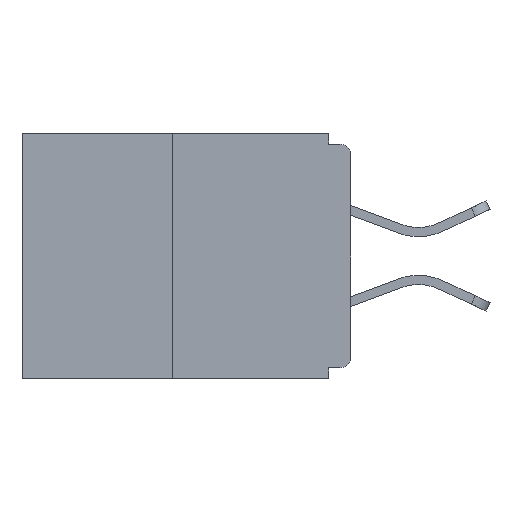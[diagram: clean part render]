
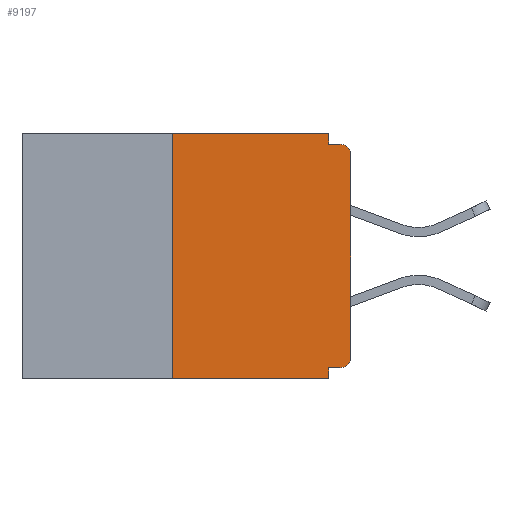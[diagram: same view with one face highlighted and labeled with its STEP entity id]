
A CAD part, left-side view. The second image highlights one B-rep face of the part: STEP entity #9197.
In plain terms, the highlighted planar face has unit normal (-1, 0, 0).
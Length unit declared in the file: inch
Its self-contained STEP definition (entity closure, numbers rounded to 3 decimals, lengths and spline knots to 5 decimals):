
#2 = VECTOR ( 'NONE', #19721, 39.37008 ) ;
#694 = DIRECTION ( 'NONE',  ( 0., 0., -1. ) ) ;
#788 = CARTESIAN_POINT ( 'NONE',  ( 0., 0.015, -0.03 ) ) ;
#896 = DIRECTION ( 'NONE',  ( 0., -1., 0. ) ) ;
#991 = VERTEX_POINT ( 'NONE', #12643 ) ;
#1147 = VERTEX_POINT ( 'NONE', #2009 ) ;
#1850 = LINE ( 'NONE', #9322, #15192 ) ;
#2009 = CARTESIAN_POINT ( 'NONE',  ( 0., 0., -0.313 ) ) ;
#2202 = VECTOR ( 'NONE', #11956, 39.37008 ) ;
#2434 = CIRCLE ( 'NONE', #19159, 0.015 ) ;
#2631 = EDGE_LOOP ( 'NONE', ( #3485, #15340, #22657, #20175, #4663, #16789, #5242, #20409, #9876, #16859 ) ) ;
#2703 = CARTESIAN_POINT ( 'NONE',  ( 0., 0., -0.015 ) ) ;
#2939 = CARTESIAN_POINT ( 'NONE',  ( 0., 0.031, -0.328 ) ) ;
#3423 = EDGE_CURVE ( 'NONE', #17848, #17363, #1850, .T. ) ;
#3485 = ORIENTED_EDGE ( 'NONE', *, *, #9588, .F. ) ;
#4242 = CIRCLE ( 'NONE', #18661, 0.015 ) ;
#4546 = VECTOR ( 'NONE', #11085, 39.37008 ) ;
#4663 = ORIENTED_EDGE ( 'NONE', *, *, #13185, .F. ) ;
#5237 = EDGE_CURVE ( 'NONE', #8949, #17363, #11205, .T. ) ;
#5242 = ORIENTED_EDGE ( 'NONE', *, *, #16992, .T. ) ;
#5782 = LINE ( 'NONE', #10197, #16762 ) ;
#6923 = VECTOR ( 'NONE', #18237, 39.37008 ) ;
#6983 = DIRECTION ( 'NONE',  ( 0., 1., 0. ) ) ;
#7072 = VERTEX_POINT ( 'NONE', #23327 ) ;
#7224 = LINE ( 'NONE', #10923, #19122 ) ;
#7410 = EDGE_CURVE ( 'NONE', #7072, #12155, #2434, .T. ) ;
#7433 = CARTESIAN_POINT ( 'NONE',  ( 0., 0.25, 0. ) ) ;
#8226 = DIRECTION ( 'NONE',  ( -1., 0., 0. ) ) ;
#8374 = CARTESIAN_POINT ( 'NONE',  ( 0., 0.46, 0. ) ) ;
#8459 = EDGE_CURVE ( 'NONE', #991, #12155, #19389, .T. ) ;
#8869 = EDGE_CURVE ( 'NONE', #16412, #1147, #4242, .T. ) ;
#8911 = EDGE_CURVE ( 'NONE', #8949, #9071, #23619, .T. ) ;
#8949 = VERTEX_POINT ( 'NONE', #10281 ) ;
#9071 = VERTEX_POINT ( 'NONE', #7433 ) ;
#9197 = ADVANCED_FACE ( 'NONE', ( #17611 ), #13836, .F. ) ;
#9322 = CARTESIAN_POINT ( 'NONE',  ( 0., 0.031, -0.343 ) ) ;
#9373 = LINE ( 'NONE', #12889, #6923 ) ;
#9588 = EDGE_CURVE ( 'NONE', #9071, #14831, #5782, .T. ) ;
#9646 = CARTESIAN_POINT ( 'NONE',  ( 0., 0.031, -0.343 ) ) ;
#9876 = ORIENTED_EDGE ( 'NONE', *, *, #8459, .F. ) ;
#9958 = DIRECTION ( 'NONE',  ( 0., -1., 0. ) ) ;
#10197 = CARTESIAN_POINT ( 'NONE',  ( 0., 0.46, 0. ) ) ;
#10281 = CARTESIAN_POINT ( 'NONE',  ( 0., 0.25, -0.343 ) ) ;
#10387 = CARTESIAN_POINT ( 'NONE',  ( 0., 0., 0. ) ) ;
#10553 = AXIS2_PLACEMENT_3D ( 'NONE', #8374, #21355, #694 ) ;
#10923 = CARTESIAN_POINT ( 'NONE',  ( 0., 0., -0.328 ) ) ;
#11085 = DIRECTION ( 'NONE',  ( 0., -1., 0. ) ) ;
#11205 = LINE ( 'NONE', #13130, #4546 ) ;
#11379 = DIRECTION ( 'NONE',  ( 0., 0., -1. ) ) ;
#11956 = DIRECTION ( 'NONE',  ( 0., 0., 1. ) ) ;
#12044 = VECTOR ( 'NONE', #896, 39.37008 ) ;
#12155 = VERTEX_POINT ( 'NONE', #18155 ) ;
#12643 = CARTESIAN_POINT ( 'NONE',  ( 0., 0.031, -0.015 ) ) ;
#12889 = CARTESIAN_POINT ( 'NONE',  ( 0., 0.031, 0. ) ) ;
#13130 = CARTESIAN_POINT ( 'NONE',  ( 0., 0.46, -0.343 ) ) ;
#13185 = EDGE_CURVE ( 'NONE', #16412, #17848, #7224, .T. ) ;
#13420 = CARTESIAN_POINT ( 'NONE',  ( 0., 0.015, -0.313 ) ) ;
#13836 = PLANE ( 'NONE',  #10553 ) ;
#14831 = VERTEX_POINT ( 'NONE', #22375 ) ;
#15192 = VECTOR ( 'NONE', #11379, 39.37008 ) ;
#15340 = ORIENTED_EDGE ( 'NONE', *, *, #8911, .F. ) ;
#15631 = DIRECTION ( 'NONE',  ( 0., 0., -1. ) ) ;
#16412 = VERTEX_POINT ( 'NONE', #22533 ) ;
#16762 = VECTOR ( 'NONE', #9958, 39.37008 ) ;
#16789 = ORIENTED_EDGE ( 'NONE', *, *, #8869, .T. ) ;
#16859 = ORIENTED_EDGE ( 'NONE', *, *, #18218, .F. ) ;
#16992 = EDGE_CURVE ( 'NONE', #1147, #7072, #21155, .T. ) ;
#17363 = VERTEX_POINT ( 'NONE', #9646 ) ;
#17611 = FACE_OUTER_BOUND ( 'NONE', #2631, .T. ) ;
#17848 = VERTEX_POINT ( 'NONE', #2939 ) ;
#18155 = CARTESIAN_POINT ( 'NONE',  ( 0., 0.015, -0.015 ) ) ;
#18218 = EDGE_CURVE ( 'NONE', #14831, #991, #9373, .T. ) ;
#18237 = DIRECTION ( 'NONE',  ( 0., 0., -1. ) ) ;
#18661 = AXIS2_PLACEMENT_3D ( 'NONE', #13420, #20813, #19008 ) ;
#19008 = DIRECTION ( 'NONE',  ( 0., 0., -1. ) ) ;
#19122 = VECTOR ( 'NONE', #6983, 39.37008 ) ;
#19159 = AXIS2_PLACEMENT_3D ( 'NONE', #788, #8226, #15631 ) ;
#19389 = LINE ( 'NONE', #2703, #12044 ) ;
#19721 = DIRECTION ( 'NONE',  ( 0., 0., 1. ) ) ;
#20175 = ORIENTED_EDGE ( 'NONE', *, *, #3423, .F. ) ;
#20409 = ORIENTED_EDGE ( 'NONE', *, *, #7410, .T. ) ;
#20813 = DIRECTION ( 'NONE',  ( -1., 0., 0. ) ) ;
#21155 = LINE ( 'NONE', #10387, #2202 ) ;
#21355 = DIRECTION ( 'NONE',  ( 1., 0., 0. ) ) ;
#22375 = CARTESIAN_POINT ( 'NONE',  ( 0., 0.031, 0. ) ) ;
#22533 = CARTESIAN_POINT ( 'NONE',  ( 0., 0.015, -0.328 ) ) ;
#22657 = ORIENTED_EDGE ( 'NONE', *, *, #5237, .T. ) ;
#23250 = CARTESIAN_POINT ( 'NONE',  ( 0., 0.25, 0. ) ) ;
#23327 = CARTESIAN_POINT ( 'NONE',  ( 0., 0., -0.03 ) ) ;
#23619 = LINE ( 'NONE', #23250, #2 ) ;
